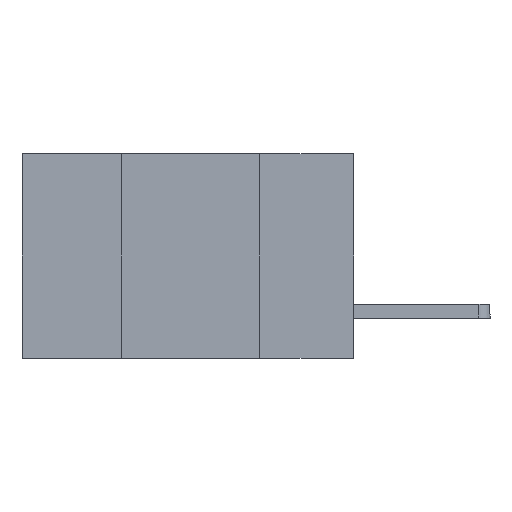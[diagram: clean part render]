
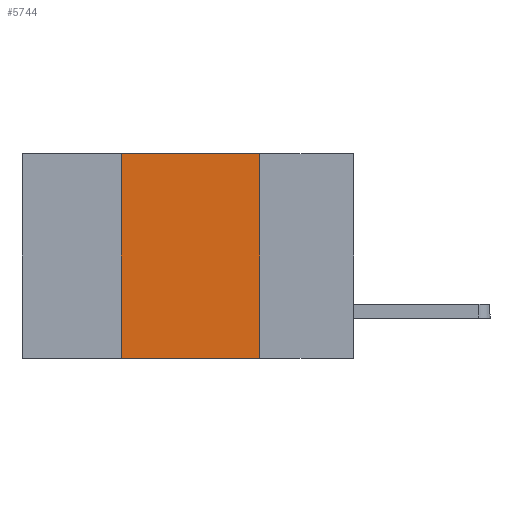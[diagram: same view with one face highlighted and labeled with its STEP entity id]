
A CAD part, left-side view. The second image highlights one B-rep face of the part: STEP entity #5744.
In plain terms, the highlighted planar face has unit normal (-1, 0, 0).
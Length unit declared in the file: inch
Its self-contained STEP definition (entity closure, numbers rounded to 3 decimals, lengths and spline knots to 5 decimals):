
#173 = DIRECTION ( 'NONE',  ( 0., 0., 1. ) ) ;
#715 = CARTESIAN_POINT ( 'NONE',  ( 0., 0.42, 0. ) ) ;
#1117 = CARTESIAN_POINT ( 'NONE',  ( 0., 0.17, -0.37 ) ) ;
#1481 = VERTEX_POINT ( 'NONE', #715 ) ;
#1525 = ORIENTED_EDGE ( 'NONE', *, *, #4829, .F. ) ;
#1919 = PLANE ( 'NONE',  #3728 ) ;
#2708 = VERTEX_POINT ( 'NONE', #1117 ) ;
#3369 = ORIENTED_EDGE ( 'NONE', *, *, #12834, .T. ) ;
#3728 = AXIS2_PLACEMENT_3D ( 'NONE', #12334, #13339, #7341 ) ;
#4076 = CARTESIAN_POINT ( 'NONE',  ( 0., 0.6, -0.37 ) ) ;
#4155 = CARTESIAN_POINT ( 'NONE',  ( 0., 0.17, 0. ) ) ;
#4310 = VECTOR ( 'NONE', #7076, 39.37008 ) ;
#4483 = LINE ( 'NONE', #4076, #6933 ) ;
#4582 = ORIENTED_EDGE ( 'NONE', *, *, #11155, .F. ) ;
#4829 = EDGE_CURVE ( 'NONE', #13624, #1481, #13542, .T. ) ;
#4990 = LINE ( 'NONE', #12058, #4310 ) ;
#5270 = ORIENTED_EDGE ( 'NONE', *, *, #12719, .F. ) ;
#5744 = ADVANCED_FACE ( 'NONE', ( #13209 ), #1919, .F. ) ;
#5859 = LINE ( 'NONE', #4155, #11523 ) ;
#6885 = CARTESIAN_POINT ( 'NONE',  ( 0., 0.42, 0. ) ) ;
#6933 = VECTOR ( 'NONE', #13187, 39.37008 ) ;
#7076 = DIRECTION ( 'NONE',  ( 0., -1., 0. ) ) ;
#7341 = DIRECTION ( 'NONE',  ( 0., 0., -1. ) ) ;
#8550 = CARTESIAN_POINT ( 'NONE',  ( 0., 0.17, 0. ) ) ;
#8562 = VECTOR ( 'NONE', #173, 39.37008 ) ;
#9780 = EDGE_LOOP ( 'NONE', ( #4582, #5270, #1525, #3369 ) ) ;
#11155 = EDGE_CURVE ( 'NONE', #13626, #2708, #5859, .T. ) ;
#11523 = VECTOR ( 'NONE', #12300, 39.37008 ) ;
#12058 = CARTESIAN_POINT ( 'NONE',  ( 0., 0.6, 0. ) ) ;
#12300 = DIRECTION ( 'NONE',  ( 0., 0., -1. ) ) ;
#12334 = CARTESIAN_POINT ( 'NONE',  ( 0., 0.6, 0. ) ) ;
#12719 = EDGE_CURVE ( 'NONE', #1481, #13626, #4990, .T. ) ;
#12834 = EDGE_CURVE ( 'NONE', #13624, #2708, #4483, .T. ) ;
#13187 = DIRECTION ( 'NONE',  ( 0., -1., 0. ) ) ;
#13209 = FACE_OUTER_BOUND ( 'NONE', #9780, .T. ) ;
#13339 = DIRECTION ( 'NONE',  ( 1., 0., 0. ) ) ;
#13512 = CARTESIAN_POINT ( 'NONE',  ( 0., 0.42, -0.37 ) ) ;
#13542 = LINE ( 'NONE', #6885, #8562 ) ;
#13624 = VERTEX_POINT ( 'NONE', #13512 ) ;
#13626 = VERTEX_POINT ( 'NONE', #8550 ) ;
